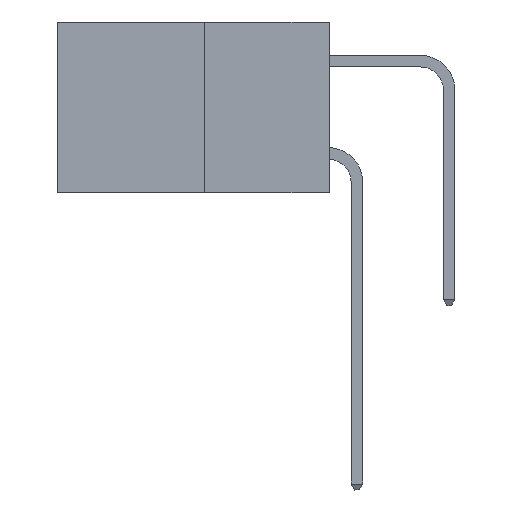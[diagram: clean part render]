
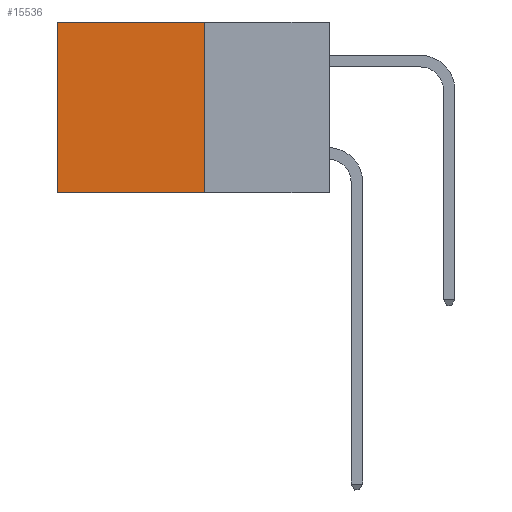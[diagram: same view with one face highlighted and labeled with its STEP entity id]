
A CAD part, left-side view. The second image highlights one B-rep face of the part: STEP entity #15536.
In plain terms, the highlighted planar face has unit normal (-1, 0, 0).
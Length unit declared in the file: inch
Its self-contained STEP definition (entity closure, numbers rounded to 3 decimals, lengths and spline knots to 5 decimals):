
#325 = VERTEX_POINT ( 'NONE', #17489 ) ;
#637 = EDGE_CURVE ( 'NONE', #2946, #15962, #18093, .T. ) ;
#1324 = VECTOR ( 'NONE', #23691, 39.37008 ) ;
#1893 = ORIENTED_EDGE ( 'NONE', *, *, #15372, .T. ) ;
#2946 = VERTEX_POINT ( 'NONE', #3040 ) ;
#3040 = CARTESIAN_POINT ( 'NONE',  ( 0.277, 0.27, -0.37 ) ) ;
#3585 = FACE_OUTER_BOUND ( 'NONE', #10503, .T. ) ;
#3799 = LINE ( 'NONE', #23651, #21183 ) ;
#3971 = CARTESIAN_POINT ( 'NONE',  ( 0.277, 0.27, 0. ) ) ;
#4444 = PLANE ( 'NONE',  #17765 ) ;
#4535 = CARTESIAN_POINT ( 'NONE',  ( 0.277, 0.59, -0.37 ) ) ;
#6092 = VERTEX_POINT ( 'NONE', #22383 ) ;
#6681 = DIRECTION ( 'NONE',  ( 0., 0., -1. ) ) ;
#6703 = ORIENTED_EDGE ( 'NONE', *, *, #637, .F. ) ;
#6967 = VECTOR ( 'NONE', #16502, 39.37008 ) ;
#7475 = VECTOR ( 'NONE', #6681, 39.37008 ) ;
#8756 = DIRECTION ( 'NONE',  ( 0., 0., -1. ) ) ;
#9143 = DIRECTION ( 'NONE',  ( 0., 0., -1. ) ) ;
#10503 = EDGE_LOOP ( 'NONE', ( #18184, #6703, #13333, #1893 ) ) ;
#13333 = ORIENTED_EDGE ( 'NONE', *, *, #20084, .F. ) ;
#15372 = EDGE_CURVE ( 'NONE', #6092, #325, #18692, .T. ) ;
#15536 = ADVANCED_FACE ( 'NONE', ( #3585 ), #4444, .F. ) ;
#15962 = VERTEX_POINT ( 'NONE', #22512 ) ;
#16502 = DIRECTION ( 'NONE',  ( 0., 1., 0. ) ) ;
#17489 = CARTESIAN_POINT ( 'NONE',  ( 0.277, 0.59, 0. ) ) ;
#17765 = AXIS2_PLACEMENT_3D ( 'NONE', #19081, #21192, #8756 ) ;
#18093 = LINE ( 'NONE', #24474, #1324 ) ;
#18184 = ORIENTED_EDGE ( 'NONE', *, *, #20607, .T. ) ;
#18692 = LINE ( 'NONE', #3971, #6967 ) ;
#19081 = CARTESIAN_POINT ( 'NONE',  ( 0.277, 0.27, -0.37 ) ) ;
#20084 = EDGE_CURVE ( 'NONE', #6092, #2946, #3799, .T. ) ;
#20607 = EDGE_CURVE ( 'NONE', #325, #15962, #24070, .T. ) ;
#21183 = VECTOR ( 'NONE', #9143, 39.37008 ) ;
#21192 = DIRECTION ( 'NONE',  ( 1., 0., 0. ) ) ;
#22383 = CARTESIAN_POINT ( 'NONE',  ( 0.277, 0.27, 0. ) ) ;
#22512 = CARTESIAN_POINT ( 'NONE',  ( 0.277, 0.59, -0.37 ) ) ;
#23651 = CARTESIAN_POINT ( 'NONE',  ( 0.277, 0.27, -0.37 ) ) ;
#23691 = DIRECTION ( 'NONE',  ( 0., 1., 0. ) ) ;
#24070 = LINE ( 'NONE', #4535, #7475 ) ;
#24474 = CARTESIAN_POINT ( 'NONE',  ( 0.277, 0.27, -0.37 ) ) ;
